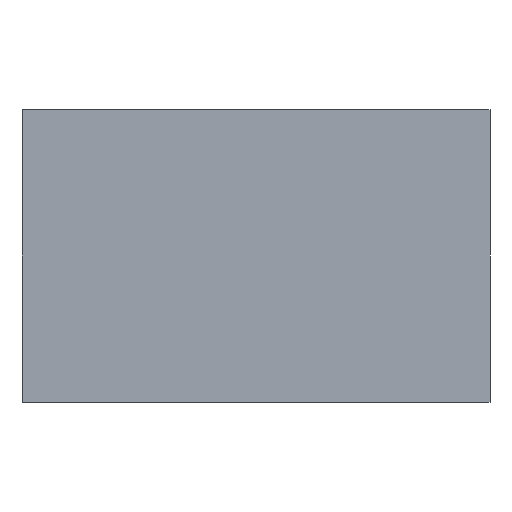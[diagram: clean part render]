
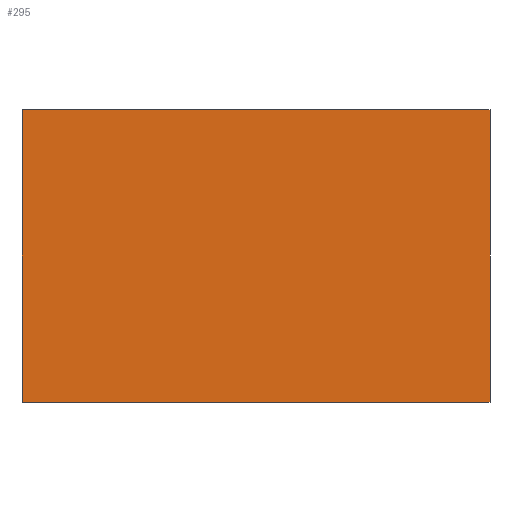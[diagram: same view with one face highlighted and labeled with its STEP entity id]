
A CAD part, front view. The second image highlights one B-rep face of the part: STEP entity #295.
In plain terms, the highlighted planar face has unit normal (0, -1, 0).
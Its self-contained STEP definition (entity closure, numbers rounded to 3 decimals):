
#13 = LINE ( 'NONE', #333, #22 ) ;
#19 = PLANE ( 'NONE',  #292 ) ;
#22 = VECTOR ( 'NONE', #26, 1000. ) ;
#26 = DIRECTION ( 'NONE',  ( -1., 0., 0. ) ) ;
#32 = VECTOR ( 'NONE', #160, 1000. ) ;
#35 = CARTESIAN_POINT ( 'NONE',  ( 15.851, 33.194, 5. ) ) ;
#36 = DIRECTION ( 'NONE',  ( 0., -1., 0. ) ) ;
#38 = DIRECTION ( 'NONE',  ( 0., 0., -1. ) ) ;
#42 = VECTOR ( 'NONE', #130, 1000. ) ;
#43 = FACE_OUTER_BOUND ( 'NONE', #328, .T. ) ;
#44 = LINE ( 'NONE', #132, #42 ) ;
#59 = EDGE_CURVE ( 'NONE', #170, #207, #44, .T. ) ;
#69 = LINE ( 'NONE', #258, #32 ) ;
#72 = EDGE_CURVE ( 'NONE', #241, #122, #69, .T. ) ;
#99 = CARTESIAN_POINT ( 'NONE',  ( 15.851, 33.194, 5. ) ) ;
#100 = DIRECTION ( 'NONE',  ( -1., 0., 0. ) ) ;
#107 = CARTESIAN_POINT ( 'NONE',  ( 7.851, 33.194, 5. ) ) ;
#122 = VERTEX_POINT ( 'NONE', #213 ) ;
#130 = DIRECTION ( 'NONE',  ( 0., 0., -1. ) ) ;
#132 = CARTESIAN_POINT ( 'NONE',  ( 15.851, 33.194, 5. ) ) ;
#148 = EDGE_CURVE ( 'NONE', #207, #122, #13, .T. ) ;
#149 = ORIENTED_EDGE ( 'NONE', *, *, #59, .F. ) ;
#150 = ORIENTED_EDGE ( 'NONE', *, *, #72, .T. ) ;
#153 = ORIENTED_EDGE ( 'NONE', *, *, #303, .T. ) ;
#160 = DIRECTION ( 'NONE',  ( 0., 0., -1. ) ) ;
#170 = VERTEX_POINT ( 'NONE', #335 ) ;
#200 = ORIENTED_EDGE ( 'NONE', *, *, #148, .F. ) ;
#207 = VERTEX_POINT ( 'NONE', #249 ) ;
#213 = CARTESIAN_POINT ( 'NONE',  ( 7.851, 33.194, 0. ) ) ;
#241 = VERTEX_POINT ( 'NONE', #107 ) ;
#249 = CARTESIAN_POINT ( 'NONE',  ( 15.851, 33.194, 0. ) ) ;
#258 = CARTESIAN_POINT ( 'NONE',  ( 7.851, 33.194, 5. ) ) ;
#272 = VECTOR ( 'NONE', #100, 1000. ) ;
#292 = AXIS2_PLACEMENT_3D ( 'NONE', #35, #36, #38 ) ;
#295 = ADVANCED_FACE ( 'NONE', ( #43 ), #19, .T. ) ;
#303 = EDGE_CURVE ( 'NONE', #170, #241, #334, .T. ) ;
#328 = EDGE_LOOP ( 'NONE', ( #200, #149, #153, #150 ) ) ;
#333 = CARTESIAN_POINT ( 'NONE',  ( 15.851, 33.194, 0. ) ) ;
#334 = LINE ( 'NONE', #99, #272 ) ;
#335 = CARTESIAN_POINT ( 'NONE',  ( 15.851, 33.194, 5. ) ) ;
